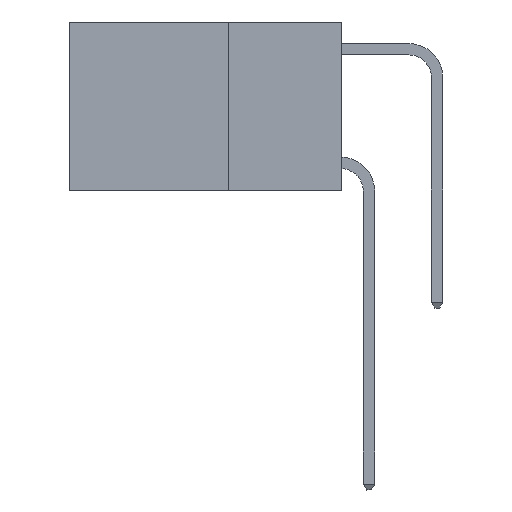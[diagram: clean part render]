
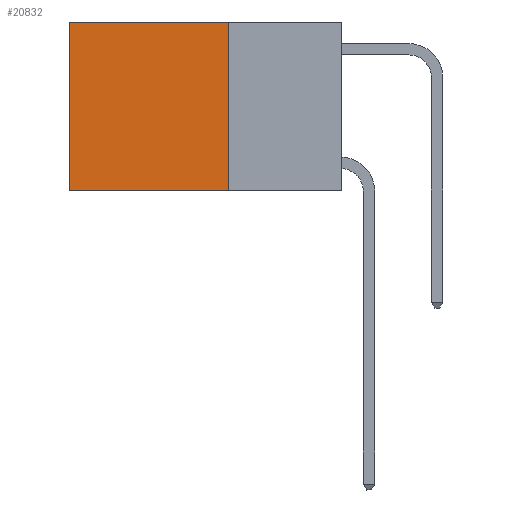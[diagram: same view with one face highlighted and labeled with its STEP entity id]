
A CAD part, left-side view. The second image highlights one B-rep face of the part: STEP entity #20832.
In plain terms, the highlighted planar face has unit normal (-1, 0, 0).
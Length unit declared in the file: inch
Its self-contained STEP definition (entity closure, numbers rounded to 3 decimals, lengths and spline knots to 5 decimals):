
#235 = CARTESIAN_POINT ( 'NONE',  ( 0.2625, 0.25, -0.37 ) ) ;
#359 = VERTEX_POINT ( 'NONE', #11934 ) ;
#533 = AXIS2_PLACEMENT_3D ( 'NONE', #4916, #5041, #10358 ) ;
#615 = ORIENTED_EDGE ( 'NONE', *, *, #1821, .F. ) ;
#1821 = EDGE_CURVE ( 'NONE', #20128, #18486, #14650, .T. ) ;
#4070 = CARTESIAN_POINT ( 'NONE',  ( 0.2625, 0.25, 0. ) ) ;
#4301 = CARTESIAN_POINT ( 'NONE',  ( 0.2625, 0.6, -0.37 ) ) ;
#4916 = CARTESIAN_POINT ( 'NONE',  ( 0.2625, 0.25, 0. ) ) ;
#5041 = DIRECTION ( 'NONE',  ( 1., 0., 0. ) ) ;
#5120 = LINE ( 'NONE', #235, #6614 ) ;
#5885 = EDGE_CURVE ( 'NONE', #359, #9067, #13519, .T. ) ;
#6169 = VECTOR ( 'NONE', #20619, 39.37008 ) ;
#6270 = ORIENTED_EDGE ( 'NONE', *, *, #19239, .T. ) ;
#6614 = VECTOR ( 'NONE', #15349, 39.37008 ) ;
#6940 = FACE_OUTER_BOUND ( 'NONE', #15251, .T. ) ;
#7554 = DIRECTION ( 'NONE',  ( 0., 1., 0. ) ) ;
#8029 = VECTOR ( 'NONE', #7554, 39.37008 ) ;
#9067 = VERTEX_POINT ( 'NONE', #4301 ) ;
#10358 = DIRECTION ( 'NONE',  ( 0., 0., -1. ) ) ;
#10864 = LINE ( 'NONE', #14611, #8029 ) ;
#11934 = CARTESIAN_POINT ( 'NONE',  ( 0.2625, 0.6, 0. ) ) ;
#12024 = CARTESIAN_POINT ( 'NONE',  ( 0.2625, 0.6, 0. ) ) ;
#12983 = DIRECTION ( 'NONE',  ( 0., 0., -1. ) ) ;
#13519 = LINE ( 'NONE', #12024, #6169 ) ;
#14611 = CARTESIAN_POINT ( 'NONE',  ( 0.2625, 0.25, 0. ) ) ;
#14650 = LINE ( 'NONE', #4070, #20066 ) ;
#15251 = EDGE_LOOP ( 'NONE', ( #20574, #16138, #615, #6270 ) ) ;
#15349 = DIRECTION ( 'NONE',  ( 0., 1., 0. ) ) ;
#15610 = PLANE ( 'NONE',  #533 ) ;
#15818 = EDGE_CURVE ( 'NONE', #18486, #9067, #5120, .T. ) ;
#16138 = ORIENTED_EDGE ( 'NONE', *, *, #15818, .F. ) ;
#18486 = VERTEX_POINT ( 'NONE', #19874 ) ;
#19239 = EDGE_CURVE ( 'NONE', #20128, #359, #10864, .T. ) ;
#19874 = CARTESIAN_POINT ( 'NONE',  ( 0.2625, 0.25, -0.37 ) ) ;
#20066 = VECTOR ( 'NONE', #12983, 39.37008 ) ;
#20128 = VERTEX_POINT ( 'NONE', #21299 ) ;
#20574 = ORIENTED_EDGE ( 'NONE', *, *, #5885, .T. ) ;
#20619 = DIRECTION ( 'NONE',  ( 0., 0., -1. ) ) ;
#20832 = ADVANCED_FACE ( 'NONE', ( #6940 ), #15610, .F. ) ;
#21299 = CARTESIAN_POINT ( 'NONE',  ( 0.2625, 0.25, 0. ) ) ;
